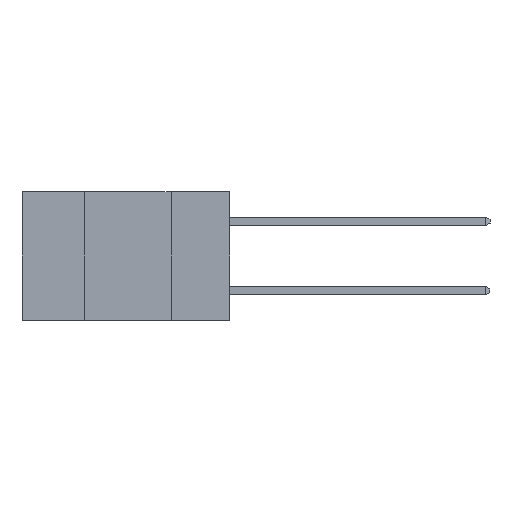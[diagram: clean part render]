
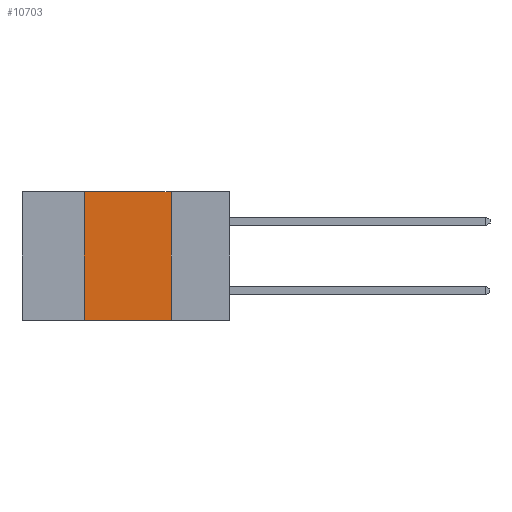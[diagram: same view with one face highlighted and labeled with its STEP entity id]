
A CAD part, left-side view. The second image highlights one B-rep face of the part: STEP entity #10703.
In plain terms, the highlighted planar face has unit normal (-1, 0, 0).
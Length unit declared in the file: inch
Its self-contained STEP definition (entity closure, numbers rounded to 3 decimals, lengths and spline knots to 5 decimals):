
#5 = DIRECTION ( 'NONE',  ( 0., -1., 0. ) ) ;
#567 = FACE_OUTER_BOUND ( 'NONE', #1064, .T. ) ;
#666 = DIRECTION ( 'NONE',  ( 0., -1., 0. ) ) ;
#1015 = CARTESIAN_POINT ( 'NONE',  ( 0., 0.17, 0. ) ) ;
#1064 = EDGE_LOOP ( 'NONE', ( #2803, #11379, #7558, #4649 ) ) ;
#2803 = ORIENTED_EDGE ( 'NONE', *, *, #8991, .F. ) ;
#3724 = EDGE_CURVE ( 'NONE', #8352, #9921, #8459, .T. ) ;
#3902 = DIRECTION ( 'NONE',  ( 1., 0., 0. ) ) ;
#4222 = LINE ( 'NONE', #8473, #11183 ) ;
#4649 = ORIENTED_EDGE ( 'NONE', *, *, #4924, .T. ) ;
#4799 = CARTESIAN_POINT ( 'NONE',  ( 0., 0.17, -0.37 ) ) ;
#4924 = EDGE_CURVE ( 'NONE', #8352, #8931, #4222, .T. ) ;
#5507 = VECTOR ( 'NONE', #12708, 39.37008 ) ;
#5906 = DIRECTION ( 'NONE',  ( 0., 0., 1. ) ) ;
#6312 = LINE ( 'NONE', #1015, #5507 ) ;
#7558 = ORIENTED_EDGE ( 'NONE', *, *, #3724, .F. ) ;
#8147 = VECTOR ( 'NONE', #5, 39.37008 ) ;
#8150 = CARTESIAN_POINT ( 'NONE',  ( 0., 0.17, 0. ) ) ;
#8352 = VERTEX_POINT ( 'NONE', #15401 ) ;
#8442 = AXIS2_PLACEMENT_3D ( 'NONE', #11722, #3902, #13007 ) ;
#8459 = LINE ( 'NONE', #14893, #11890 ) ;
#8473 = CARTESIAN_POINT ( 'NONE',  ( 0., 0.6, -0.37 ) ) ;
#8931 = VERTEX_POINT ( 'NONE', #4799 ) ;
#8991 = EDGE_CURVE ( 'NONE', #10861, #8931, #6312, .T. ) ;
#9127 = PLANE ( 'NONE',  #8442 ) ;
#9921 = VERTEX_POINT ( 'NONE', #14120 ) ;
#10684 = EDGE_CURVE ( 'NONE', #9921, #10861, #14041, .T. ) ;
#10703 = ADVANCED_FACE ( 'NONE', ( #567 ), #9127, .F. ) ;
#10861 = VERTEX_POINT ( 'NONE', #8150 ) ;
#11183 = VECTOR ( 'NONE', #666, 39.37008 ) ;
#11379 = ORIENTED_EDGE ( 'NONE', *, *, #10684, .F. ) ;
#11722 = CARTESIAN_POINT ( 'NONE',  ( 0., 0.6, 0. ) ) ;
#11890 = VECTOR ( 'NONE', #5906, 39.37008 ) ;
#12708 = DIRECTION ( 'NONE',  ( 0., 0., -1. ) ) ;
#12958 = CARTESIAN_POINT ( 'NONE',  ( 0., 0.6, 0. ) ) ;
#13007 = DIRECTION ( 'NONE',  ( 0., 0., -1. ) ) ;
#14041 = LINE ( 'NONE', #12958, #8147 ) ;
#14120 = CARTESIAN_POINT ( 'NONE',  ( 0., 0.42, 0. ) ) ;
#14893 = CARTESIAN_POINT ( 'NONE',  ( 0., 0.42, 0. ) ) ;
#15401 = CARTESIAN_POINT ( 'NONE',  ( 0., 0.42, -0.37 ) ) ;
